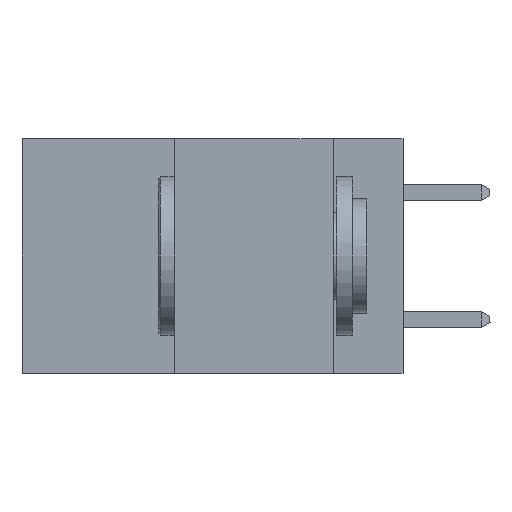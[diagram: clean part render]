
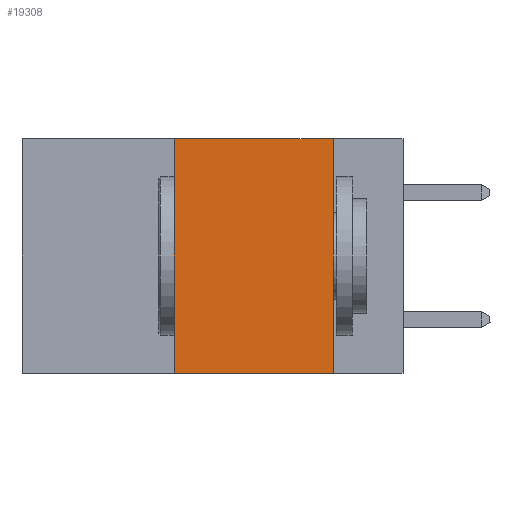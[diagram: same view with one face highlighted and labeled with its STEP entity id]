
A CAD part, left-side view. The second image highlights one B-rep face of the part: STEP entity #19308.
In plain terms, the highlighted planar face has unit normal (-1, 0, 0).
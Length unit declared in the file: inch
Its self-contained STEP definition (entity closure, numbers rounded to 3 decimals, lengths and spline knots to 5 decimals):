
#485 = CARTESIAN_POINT ( 'NONE',  ( 0., 0.36, -0.37 ) ) ;
#2430 = DIRECTION ( 'NONE',  ( 0., 0., -1. ) ) ;
#4108 = EDGE_CURVE ( 'NONE', #35286, #17207, #34949, .T. ) ;
#5946 = AXIS2_PLACEMENT_3D ( 'NONE', #17658, #30489, #15069 ) ;
#9253 = LINE ( 'NONE', #23385, #15556 ) ;
#9610 = CARTESIAN_POINT ( 'NONE',  ( 0., 0.11, -0.37 ) ) ;
#14006 = DIRECTION ( 'NONE',  ( 0., 0., 1. ) ) ;
#14498 = LINE ( 'NONE', #27374, #22299 ) ;
#14531 = PLANE ( 'NONE',  #5946 ) ;
#14985 = ORIENTED_EDGE ( 'NONE', *, *, #39692, .F. ) ;
#15069 = DIRECTION ( 'NONE',  ( 0., 0., -1. ) ) ;
#15556 = VECTOR ( 'NONE', #14006, 39.37008 ) ;
#16287 = EDGE_CURVE ( 'NONE', #21613, #28647, #27444, .T. ) ;
#16865 = DIRECTION ( 'NONE',  ( 0., -1., 0. ) ) ;
#17207 = VERTEX_POINT ( 'NONE', #40197 ) ;
#17658 = CARTESIAN_POINT ( 'NONE',  ( 0., 0.6, 0. ) ) ;
#19308 = ADVANCED_FACE ( 'NONE', ( #26726 ), #14531, .F. ) ;
#19368 = VECTOR ( 'NONE', #16865, 39.37008 ) ;
#19389 = DIRECTION ( 'NONE',  ( 0., -1., 0. ) ) ;
#21613 = VERTEX_POINT ( 'NONE', #485 ) ;
#22299 = VECTOR ( 'NONE', #2430, 39.37008 ) ;
#22651 = CARTESIAN_POINT ( 'NONE',  ( 0., 0.6, -0.37 ) ) ;
#23385 = CARTESIAN_POINT ( 'NONE',  ( 0., 0.36, 0. ) ) ;
#23774 = EDGE_CURVE ( 'NONE', #17207, #28647, #14498, .T. ) ;
#26427 = CARTESIAN_POINT ( 'NONE',  ( 0., 0.6, 0. ) ) ;
#26726 = FACE_OUTER_BOUND ( 'NONE', #33129, .T. ) ;
#27374 = CARTESIAN_POINT ( 'NONE',  ( 0., 0.11, 0. ) ) ;
#27444 = LINE ( 'NONE', #22651, #34267 ) ;
#27602 = ORIENTED_EDGE ( 'NONE', *, *, #16287, .T. ) ;
#28647 = VERTEX_POINT ( 'NONE', #9610 ) ;
#29854 = CARTESIAN_POINT ( 'NONE',  ( 0., 0.36, 0. ) ) ;
#30489 = DIRECTION ( 'NONE',  ( 1., 0., 0. ) ) ;
#33129 = EDGE_LOOP ( 'NONE', ( #37431, #38413, #14985, #27602 ) ) ;
#34267 = VECTOR ( 'NONE', #19389, 39.37008 ) ;
#34949 = LINE ( 'NONE', #26427, #19368 ) ;
#35286 = VERTEX_POINT ( 'NONE', #29854 ) ;
#37431 = ORIENTED_EDGE ( 'NONE', *, *, #23774, .F. ) ;
#38413 = ORIENTED_EDGE ( 'NONE', *, *, #4108, .F. ) ;
#39692 = EDGE_CURVE ( 'NONE', #21613, #35286, #9253, .T. ) ;
#40197 = CARTESIAN_POINT ( 'NONE',  ( 0., 0.11, 0. ) ) ;
